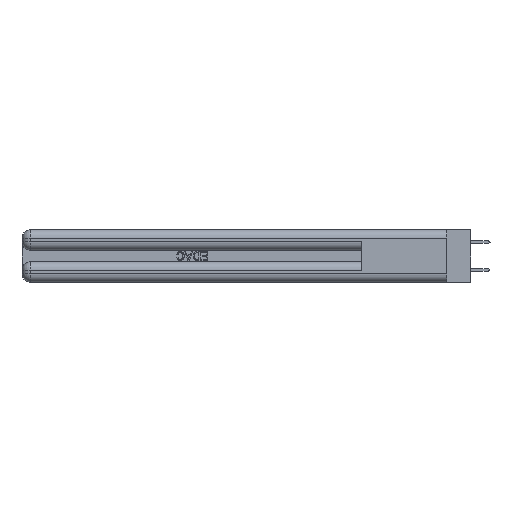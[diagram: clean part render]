
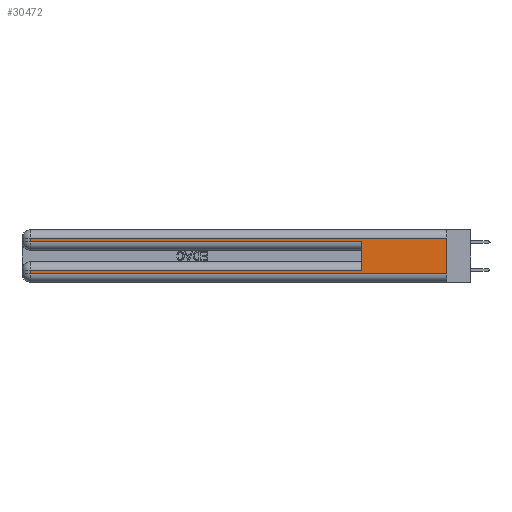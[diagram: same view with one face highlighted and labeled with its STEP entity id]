
A CAD part, left-side view. The second image highlights one B-rep face of the part: STEP entity #30472.
In plain terms, the highlighted planar face has unit normal (-1, 0, 0).
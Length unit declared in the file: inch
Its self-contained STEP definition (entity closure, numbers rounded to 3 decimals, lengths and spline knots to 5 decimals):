
#25 = LINE ( 'NONE', #3034, #22543 ) ;
#618 = LINE ( 'NONE', #16694, #23715 ) ;
#828 = CARTESIAN_POINT ( 'NONE',  ( 0., 2.94, 0.06 ) ) ;
#834 = ORIENTED_EDGE ( 'NONE', *, *, #25963, .T. ) ;
#1601 = ORIENTED_EDGE ( 'NONE', *, *, #18100, .T. ) ;
#1912 = DIRECTION ( 'NONE',  ( 0., 0., -1. ) ) ;
#3034 = CARTESIAN_POINT ( 'NONE',  ( 0., 0.6, 0.145 ) ) ;
#3722 = ORIENTED_EDGE ( 'NONE', *, *, #9021, .F. ) ;
#3748 = VECTOR ( 'NONE', #23094, 39.37008 ) ;
#4388 = PLANE ( 'NONE',  #25893 ) ;
#4677 = VERTEX_POINT ( 'NONE', #27474 ) ;
#4864 = EDGE_CURVE ( 'NONE', #47144, #48272, #25, .T. ) ;
#5264 = EDGE_CURVE ( 'NONE', #48102, #6836, #44911, .T. ) ;
#6737 = CARTESIAN_POINT ( 'NONE',  ( 0., 0., 0.37 ) ) ;
#6836 = VERTEX_POINT ( 'NONE', #27108 ) ;
#6944 = ORIENTED_EDGE ( 'NONE', *, *, #4864, .F. ) ;
#7731 = LINE ( 'NONE', #30419, #27842 ) ;
#8860 = DIRECTION ( 'NONE',  ( 1., 0., 0. ) ) ;
#9021 = EDGE_CURVE ( 'NONE', #22207, #21370, #33136, .T. ) ;
#9556 = CARTESIAN_POINT ( 'NONE',  ( 0., 0., 0.085 ) ) ;
#12655 = CARTESIAN_POINT ( 'NONE',  ( 0., 0., 0.06 ) ) ;
#16448 = VECTOR ( 'NONE', #26426, 39.37008 ) ;
#16694 = CARTESIAN_POINT ( 'NONE',  ( 0., 0., 0.285 ) ) ;
#18100 = EDGE_CURVE ( 'NONE', #6836, #48272, #618, .T. ) ;
#18524 = CARTESIAN_POINT ( 'NONE',  ( 0., 2.94, 0.37 ) ) ;
#19447 = CARTESIAN_POINT ( 'NONE',  ( 0., 0., 0.37 ) ) ;
#20843 = CARTESIAN_POINT ( 'NONE',  ( 0., 2.94, 0.31 ) ) ;
#21012 = VECTOR ( 'NONE', #30102, 39.37008 ) ;
#21318 = CARTESIAN_POINT ( 'NONE',  ( 0., 0., 0.31 ) ) ;
#21370 = VERTEX_POINT ( 'NONE', #12655 ) ;
#22207 = VERTEX_POINT ( 'NONE', #21318 ) ;
#22513 = EDGE_CURVE ( 'NONE', #22207, #48102, #7731, .T. ) ;
#22543 = VECTOR ( 'NONE', #22740, 39.37008 ) ;
#22740 = DIRECTION ( 'NONE',  ( 0., 0., 1. ) ) ;
#22937 = ORIENTED_EDGE ( 'NONE', *, *, #34415, .T. ) ;
#23094 = DIRECTION ( 'NONE',  ( 0., 0., -1. ) ) ;
#23715 = VECTOR ( 'NONE', #38138, 39.37008 ) ;
#25715 = VECTOR ( 'NONE', #39139, 39.37008 ) ;
#25893 = AXIS2_PLACEMENT_3D ( 'NONE', #19447, #8860, #1912 ) ;
#25963 = EDGE_CURVE ( 'NONE', #47144, #4677, #34706, .T. ) ;
#26426 = DIRECTION ( 'NONE',  ( 0., 0., -1. ) ) ;
#27108 = CARTESIAN_POINT ( 'NONE',  ( 0., 2.94, 0.285 ) ) ;
#27474 = CARTESIAN_POINT ( 'NONE',  ( 0., 2.94, 0.085 ) ) ;
#27842 = VECTOR ( 'NONE', #34365, 39.37008 ) ;
#29844 = DIRECTION ( 'NONE',  ( 0., -1., 0. ) ) ;
#29949 = CARTESIAN_POINT ( 'NONE',  ( 0., 0.6, 0.285 ) ) ;
#30102 = DIRECTION ( 'NONE',  ( 0., 0., -1. ) ) ;
#30419 = CARTESIAN_POINT ( 'NONE',  ( 0., 0., 0.31 ) ) ;
#30472 = ADVANCED_FACE ( 'NONE', ( #41902 ), #4388, .F. ) ;
#30561 = CARTESIAN_POINT ( 'NONE',  ( 0., 2.94, 0.37 ) ) ;
#32094 = EDGE_CURVE ( 'NONE', #43136, #21370, #36766, .T. ) ;
#32823 = CARTESIAN_POINT ( 'NONE',  ( 0., 0., 0.06 ) ) ;
#33136 = LINE ( 'NONE', #6737, #16448 ) ;
#34365 = DIRECTION ( 'NONE',  ( 0., 1., 0. ) ) ;
#34415 = EDGE_CURVE ( 'NONE', #4677, #43136, #36995, .T. ) ;
#34706 = LINE ( 'NONE', #9556, #25715 ) ;
#35298 = CARTESIAN_POINT ( 'NONE',  ( 0., 0.6, 0.085 ) ) ;
#36766 = LINE ( 'NONE', #32823, #48527 ) ;
#36995 = LINE ( 'NONE', #30561, #3748 ) ;
#37571 = EDGE_LOOP ( 'NONE', ( #3722, #46217, #41508, #1601, #6944, #834, #22937, #47506 ) ) ;
#38138 = DIRECTION ( 'NONE',  ( 0., -1., 0. ) ) ;
#39139 = DIRECTION ( 'NONE',  ( 0., 1., 0. ) ) ;
#41508 = ORIENTED_EDGE ( 'NONE', *, *, #5264, .T. ) ;
#41902 = FACE_OUTER_BOUND ( 'NONE', #37571, .T. ) ;
#43136 = VERTEX_POINT ( 'NONE', #828 ) ;
#44911 = LINE ( 'NONE', #18524, #21012 ) ;
#46217 = ORIENTED_EDGE ( 'NONE', *, *, #22513, .T. ) ;
#47144 = VERTEX_POINT ( 'NONE', #35298 ) ;
#47506 = ORIENTED_EDGE ( 'NONE', *, *, #32094, .T. ) ;
#48102 = VERTEX_POINT ( 'NONE', #20843 ) ;
#48272 = VERTEX_POINT ( 'NONE', #29949 ) ;
#48527 = VECTOR ( 'NONE', #29844, 39.37008 ) ;
